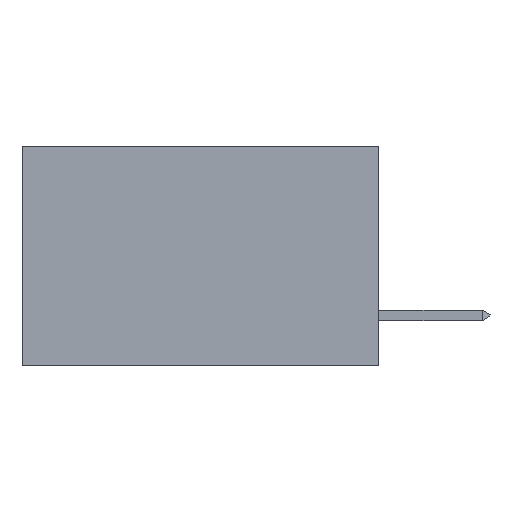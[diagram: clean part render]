
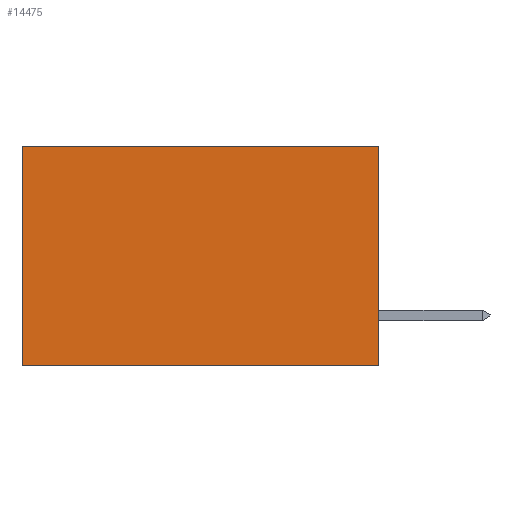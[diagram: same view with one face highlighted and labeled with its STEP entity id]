
A CAD part, left-side view. The second image highlights one B-rep face of the part: STEP entity #14475.
In plain terms, the highlighted planar face has unit normal (-1, 0, 0).
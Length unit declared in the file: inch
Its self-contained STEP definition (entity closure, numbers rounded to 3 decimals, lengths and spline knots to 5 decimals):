
#208 = CARTESIAN_POINT ( 'NONE',  ( 0.298, 0., -0.37 ) ) ;
#210 = ORIENTED_EDGE ( 'NONE', *, *, #14708, .T. ) ;
#962 = VECTOR ( 'NONE', #3362, 39.37008 ) ;
#1010 = VERTEX_POINT ( 'NONE', #6576 ) ;
#1026 = DIRECTION ( 'NONE',  ( 0., 1., 0. ) ) ;
#1359 = LINE ( 'NONE', #2103, #962 ) ;
#1544 = CARTESIAN_POINT ( 'NONE',  ( 0.298, 0., 0. ) ) ;
#1698 = ORIENTED_EDGE ( 'NONE', *, *, #2922, .F. ) ;
#2103 = CARTESIAN_POINT ( 'NONE',  ( 0.298, 0.6, 0. ) ) ;
#2503 = VECTOR ( 'NONE', #4016, 39.37008 ) ;
#2850 = EDGE_CURVE ( 'NONE', #10648, #9343, #3972, .T. ) ;
#2922 = EDGE_CURVE ( 'NONE', #1010, #10648, #14004, .T. ) ;
#3362 = DIRECTION ( 'NONE',  ( 0., 0., -1. ) ) ;
#3436 = DIRECTION ( 'NONE',  ( 1., 0., 0. ) ) ;
#3880 = FACE_OUTER_BOUND ( 'NONE', #14752, .T. ) ;
#3972 = LINE ( 'NONE', #6210, #12446 ) ;
#4016 = DIRECTION ( 'NONE',  ( 0., 1., 0. ) ) ;
#6210 = CARTESIAN_POINT ( 'NONE',  ( 0.298, 0., -0.37 ) ) ;
#6576 = CARTESIAN_POINT ( 'NONE',  ( 0.298, 0., 0. ) ) ;
#6750 = CARTESIAN_POINT ( 'NONE',  ( 0.298, 0.6, -0.37 ) ) ;
#8793 = AXIS2_PLACEMENT_3D ( 'NONE', #10873, #3436, #13538 ) ;
#9287 = VERTEX_POINT ( 'NONE', #15617 ) ;
#9343 = VERTEX_POINT ( 'NONE', #6750 ) ;
#10221 = DIRECTION ( 'NONE',  ( 0., 0., -1. ) ) ;
#10648 = VERTEX_POINT ( 'NONE', #208 ) ;
#10873 = CARTESIAN_POINT ( 'NONE',  ( 0.298, 0., 0. ) ) ;
#10973 = ORIENTED_EDGE ( 'NONE', *, *, #13179, .T. ) ;
#11089 = VECTOR ( 'NONE', #10221, 39.37008 ) ;
#12009 = ORIENTED_EDGE ( 'NONE', *, *, #2850, .F. ) ;
#12446 = VECTOR ( 'NONE', #1026, 39.37008 ) ;
#12733 = CARTESIAN_POINT ( 'NONE',  ( 0.298, 0., 0. ) ) ;
#13179 = EDGE_CURVE ( 'NONE', #9287, #9343, #1359, .T. ) ;
#13305 = PLANE ( 'NONE',  #8793 ) ;
#13538 = DIRECTION ( 'NONE',  ( 0., 0., -1. ) ) ;
#14004 = LINE ( 'NONE', #12733, #11089 ) ;
#14475 = ADVANCED_FACE ( 'NONE', ( #3880 ), #13305, .F. ) ;
#14683 = LINE ( 'NONE', #1544, #2503 ) ;
#14708 = EDGE_CURVE ( 'NONE', #1010, #9287, #14683, .T. ) ;
#14752 = EDGE_LOOP ( 'NONE', ( #10973, #12009, #1698, #210 ) ) ;
#15617 = CARTESIAN_POINT ( 'NONE',  ( 0.298, 0.6, 0. ) ) ;
